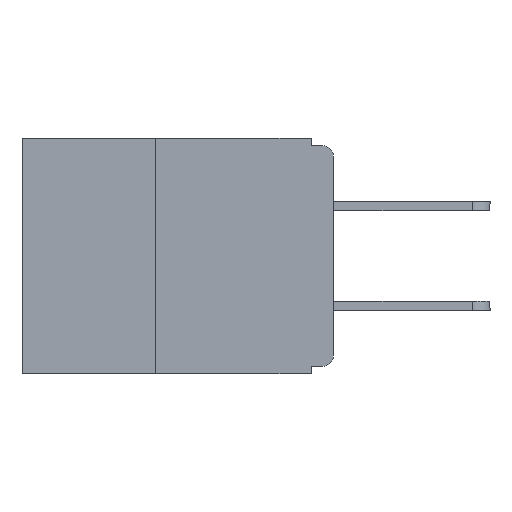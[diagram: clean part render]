
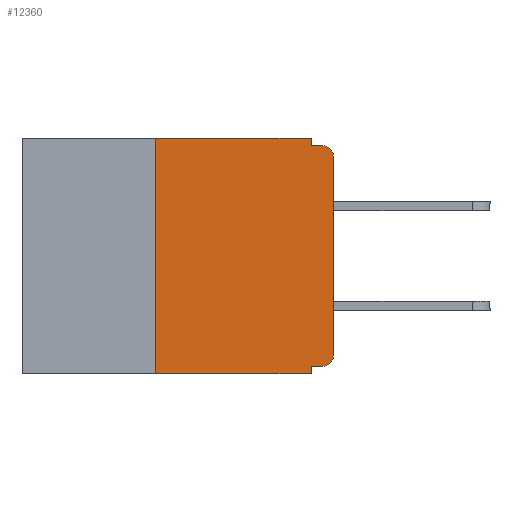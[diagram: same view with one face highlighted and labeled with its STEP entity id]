
A CAD part, left-side view. The second image highlights one B-rep face of the part: STEP entity #12360.
In plain terms, the highlighted planar face has unit normal (-1, 0, 0).
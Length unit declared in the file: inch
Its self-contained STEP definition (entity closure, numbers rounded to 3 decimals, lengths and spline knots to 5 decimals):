
#90 = LINE ( 'NONE', #2265, #442 ) ;
#217 = EDGE_CURVE ( 'NONE', #7950, #5902, #90, .T. ) ;
#261 = CARTESIAN_POINT ( 'NONE',  ( 0., 0., 0. ) ) ;
#308 = EDGE_CURVE ( 'NONE', #3763, #7950, #11196, .T. ) ;
#366 = PLANE ( 'NONE',  #10268 ) ;
#442 = VECTOR ( 'NONE', #6488, 39.37008 ) ;
#590 = EDGE_CURVE ( 'NONE', #6135, #8284, #4140, .T. ) ;
#804 = CARTESIAN_POINT ( 'NONE',  ( 0., 0.031, -0.33 ) ) ;
#816 = CARTESIAN_POINT ( 'NONE',  ( 0., 0., -0.025 ) ) ;
#1188 = CARTESIAN_POINT ( 'NONE',  ( 0., 0., -0.01 ) ) ;
#1288 = VECTOR ( 'NONE', #1858, 39.37008 ) ;
#1373 = CARTESIAN_POINT ( 'NONE',  ( 0., 0.015, -0.025 ) ) ;
#1385 = CARTESIAN_POINT ( 'NONE',  ( 0., 0.015, -0.01 ) ) ;
#1493 = CARTESIAN_POINT ( 'NONE',  ( 0., 0.437, 0. ) ) ;
#1499 = ORIENTED_EDGE ( 'NONE', *, *, #13051, .T. ) ;
#1534 = CARTESIAN_POINT ( 'NONE',  ( 0., 0.031, -0.33 ) ) ;
#1692 = ORIENTED_EDGE ( 'NONE', *, *, #6425, .T. ) ;
#1746 = CARTESIAN_POINT ( 'NONE',  ( 0., 0.031, -0.01 ) ) ;
#1805 = EDGE_CURVE ( 'NONE', #5902, #2482, #11652, .T. ) ;
#1810 = EDGE_LOOP ( 'NONE', ( #10157, #1499, #3367, #12647, #2249, #7037, #2939, #12485, #11248, #1692 ) ) ;
#1858 = DIRECTION ( 'NONE',  ( 0., 1., 0. ) ) ;
#2011 = AXIS2_PLACEMENT_3D ( 'NONE', #1373, #9138, #2485 ) ;
#2242 = DIRECTION ( 'NONE',  ( 0., 0., -1. ) ) ;
#2249 = ORIENTED_EDGE ( 'NONE', *, *, #217, .F. ) ;
#2263 = DIRECTION ( 'NONE',  ( 0., -1., 0. ) ) ;
#2265 = CARTESIAN_POINT ( 'NONE',  ( 0., 0.437, 0. ) ) ;
#2399 = VECTOR ( 'NONE', #13207, 39.37008 ) ;
#2464 = CIRCLE ( 'NONE', #2011, 0.015 ) ;
#2482 = VERTEX_POINT ( 'NONE', #1746 ) ;
#2485 = DIRECTION ( 'NONE',  ( 0., 0., -1. ) ) ;
#2616 = DIRECTION ( 'NONE',  ( 0., 0., -1. ) ) ;
#2846 = CARTESIAN_POINT ( 'NONE',  ( 0., 0.015, -0.305 ) ) ;
#2902 = EDGE_CURVE ( 'NONE', #2482, #8751, #5141, .T. ) ;
#2939 = ORIENTED_EDGE ( 'NONE', *, *, #6572, .T. ) ;
#3162 = VECTOR ( 'NONE', #8054, 39.37008 ) ;
#3181 = EDGE_CURVE ( 'NONE', #8739, #6135, #13392, .T. ) ;
#3367 = ORIENTED_EDGE ( 'NONE', *, *, #2902, .F. ) ;
#3576 = VECTOR ( 'NONE', #10693, 39.37008 ) ;
#3763 = VERTEX_POINT ( 'NONE', #10569 ) ;
#3878 = VERTEX_POINT ( 'NONE', #816 ) ;
#3986 = DIRECTION ( 'NONE',  ( 0., 0., -1. ) ) ;
#4123 = AXIS2_PLACEMENT_3D ( 'NONE', #2846, #10578, #3986 ) ;
#4140 = LINE ( 'NONE', #804, #9648 ) ;
#4147 = CARTESIAN_POINT ( 'NONE',  ( 0., 0.031, 0. ) ) ;
#4193 = CIRCLE ( 'NONE', #4123, 0.015 ) ;
#5141 = LINE ( 'NONE', #1188, #5840 ) ;
#5202 = DIRECTION ( 'NONE',  ( 0., 0., 1. ) ) ;
#5250 = CARTESIAN_POINT ( 'NONE',  ( 0., 0.25, -0.33 ) ) ;
#5600 = EDGE_CURVE ( 'NONE', #13264, #3878, #11945, .T. ) ;
#5840 = VECTOR ( 'NONE', #2263, 39.37008 ) ;
#5902 = VERTEX_POINT ( 'NONE', #4147 ) ;
#6135 = VERTEX_POINT ( 'NONE', #11159 ) ;
#6425 = EDGE_CURVE ( 'NONE', #8739, #13264, #4193, .T. ) ;
#6488 = DIRECTION ( 'NONE',  ( 0., -1., 0. ) ) ;
#6572 = EDGE_CURVE ( 'NONE', #3763, #8284, #11567, .T. ) ;
#6944 = CARTESIAN_POINT ( 'NONE',  ( 0., 0.015, -0.32 ) ) ;
#7037 = ORIENTED_EDGE ( 'NONE', *, *, #308, .F. ) ;
#7950 = VERTEX_POINT ( 'NONE', #14196 ) ;
#8054 = DIRECTION ( 'NONE',  ( 0., 0., 1. ) ) ;
#8284 = VERTEX_POINT ( 'NONE', #1534 ) ;
#8401 = CARTESIAN_POINT ( 'NONE',  ( 0., 0., -0.305 ) ) ;
#8739 = VERTEX_POINT ( 'NONE', #6944 ) ;
#8751 = VERTEX_POINT ( 'NONE', #1385 ) ;
#9138 = DIRECTION ( 'NONE',  ( -1., 0., 0. ) ) ;
#9259 = DIRECTION ( 'NONE',  ( 1., 0., 0. ) ) ;
#9648 = VECTOR ( 'NONE', #2242, 39.37008 ) ;
#10157 = ORIENTED_EDGE ( 'NONE', *, *, #5600, .T. ) ;
#10268 = AXIS2_PLACEMENT_3D ( 'NONE', #1493, #9259, #2616 ) ;
#10569 = CARTESIAN_POINT ( 'NONE',  ( 0., 0.25, -0.33 ) ) ;
#10578 = DIRECTION ( 'NONE',  ( -1., 0., 0. ) ) ;
#10677 = CARTESIAN_POINT ( 'NONE',  ( 0., 0.031, 0. ) ) ;
#10693 = DIRECTION ( 'NONE',  ( 0., 0., -1. ) ) ;
#10727 = CARTESIAN_POINT ( 'NONE',  ( 0., 0., -0.32 ) ) ;
#11148 = FACE_OUTER_BOUND ( 'NONE', #1810, .T. ) ;
#11159 = CARTESIAN_POINT ( 'NONE',  ( 0., 0.031, -0.32 ) ) ;
#11196 = LINE ( 'NONE', #5250, #13425 ) ;
#11248 = ORIENTED_EDGE ( 'NONE', *, *, #3181, .F. ) ;
#11567 = LINE ( 'NONE', #12103, #2399 ) ;
#11652 = LINE ( 'NONE', #10677, #3576 ) ;
#11945 = LINE ( 'NONE', #261, #3162 ) ;
#12103 = CARTESIAN_POINT ( 'NONE',  ( 0., 0.437, -0.33 ) ) ;
#12360 = ADVANCED_FACE ( 'NONE', ( #11148 ), #366, .F. ) ;
#12485 = ORIENTED_EDGE ( 'NONE', *, *, #590, .F. ) ;
#12647 = ORIENTED_EDGE ( 'NONE', *, *, #1805, .F. ) ;
#13051 = EDGE_CURVE ( 'NONE', #3878, #8751, #2464, .T. ) ;
#13207 = DIRECTION ( 'NONE',  ( 0., -1., 0. ) ) ;
#13264 = VERTEX_POINT ( 'NONE', #8401 ) ;
#13392 = LINE ( 'NONE', #10727, #1288 ) ;
#13425 = VECTOR ( 'NONE', #5202, 39.37008 ) ;
#14196 = CARTESIAN_POINT ( 'NONE',  ( 0., 0.25, 0. ) ) ;
